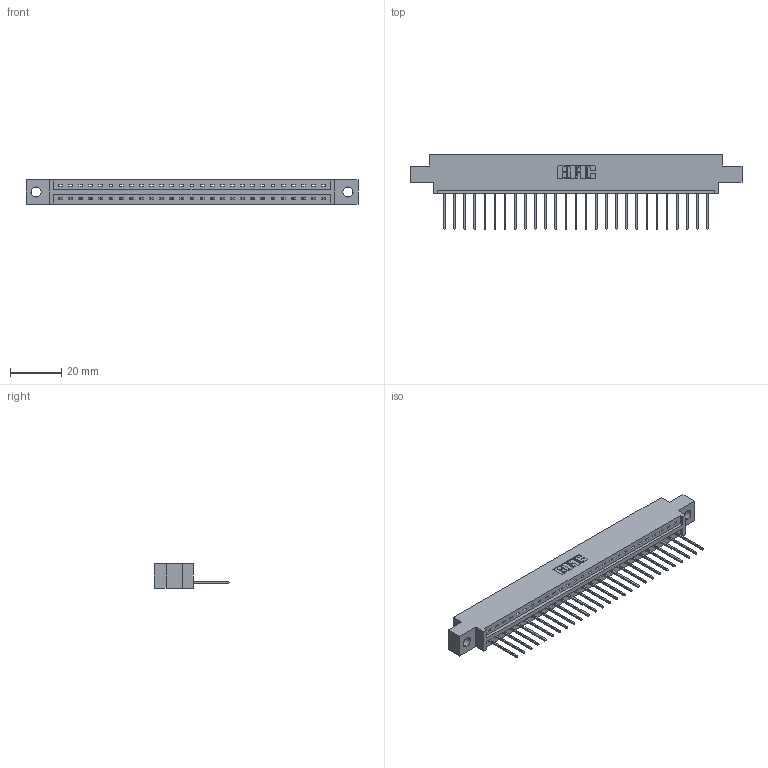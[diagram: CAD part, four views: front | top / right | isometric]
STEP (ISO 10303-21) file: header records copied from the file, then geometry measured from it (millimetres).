
FILE_DESCRIPTION (( 'STEP AP203' ), '1' );
FILE_NAME ('337-027-540-604.STEP', '2019-09-30T19:50:58', ( '' ), ( '' ), 'SwSTEP 2.0', 'SolidWorks 2016', '' );
FILE_SCHEMA (( 'CONFIG_CONTROL_DESIGN' ));
Length unit declared in the file: inch
Products named in the file (3): 337 Part_0.170 Offset - 0.156 Dia-TH; 337-027-540-604; 345-292-001_345-293-140
Assembly tree (28 placements, depth 2):
  337-027-540-604
    337 Part_0.170 Offset - 0.156 Dia-TH
    345-292-001_345-293-140  x27
Bounding box: 130 x 29.47 x 9.4 mm (x, y, z)
Volume: 13154.5 mm3; surface area: 13673.1 mm2
Topology: 28 solids, 28 shells, 1792 faces, 5399 edges, 3562 vertices
Faces by surface type: plane 1316, cylinder 476
Entity records: 22163 total; most frequent: CARTESIAN_POINT 3867, ORIENTED_EDGE 3830, DIRECTION 3285, EDGE_CURVE 1915, VECTOR 1787, LINE 1787, VERTEX_POINT 1274, AXIS2_PLACEMENT_3D 749
